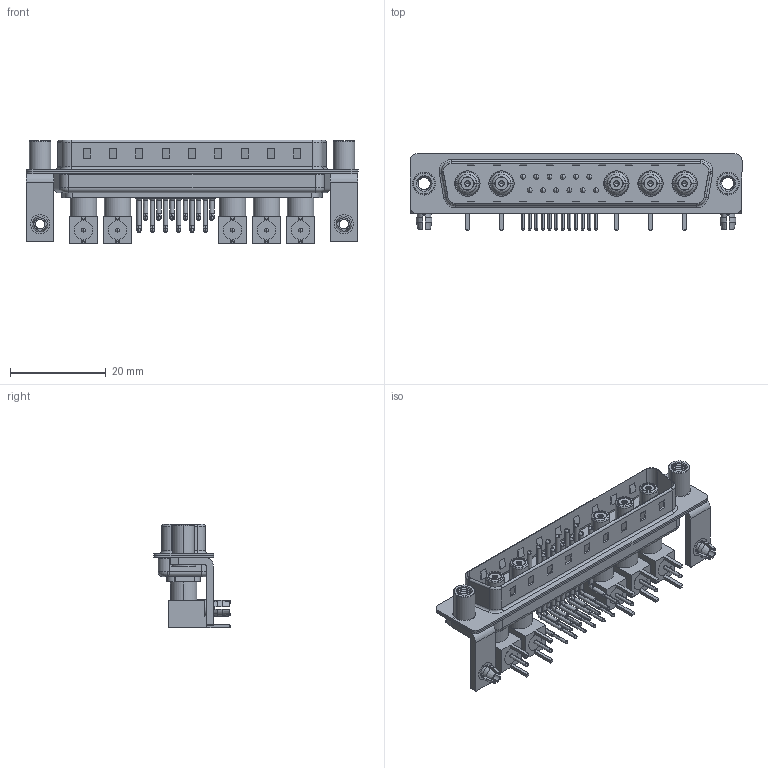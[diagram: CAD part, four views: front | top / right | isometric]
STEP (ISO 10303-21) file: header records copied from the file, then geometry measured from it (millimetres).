
FILE_DESCRIPTION (( 'STEP AP203' ), '1' );
FILE_NAME ('629-17W5240-7ND.STEP', '2022-05-15T00:04:30', ( '' ), ( '' ), 'SwSTEP 2.0', 'SolidWorks 2020', '' );
FILE_SCHEMA (( 'CONFIG_CONTROL_DESIGN' ));
Length unit declared in the file: millimetre
Products named in the file (21): 629Combo Stabilizer Bracket; 629Combo Contact Row 2; 629Combo Shell Front_37 Contacts; Socket_RA; Insulator RA Pin; 629-17W5240-7ND; Co-Ax Jack Assy_RA; Insulator Socket; 629Combo Threaded Standoff_D; Co-Ax Jack_RA PC Tail; 629Combo Housing_17W5; 629Combo Contact Row 1; Locking Collar; 629Combo Shell Rear_37 Contacts; 629Combo Board Lock; RA Back Shell; Insulator Socket 2
Assembly tree (61 placements, depth 3):
  629-17W5240-7ND
    629Combo Housing_17W5
    629Combo Shell Rear_37 Contacts
    629Combo Shell Front_37 Contacts
    629Combo Stabilizer Bracket  x2
    629Combo Board Lock  x2
    629Combo Threaded Standoff_D  x2
    Co-Ax Jack Assy_RA
      Co-Ax Jack_RA PC Tail
      Insulator Socket
      Insulator Socket 2
      Locking Collar
      Socket_RA
      RA Back Shell
      Insulator RA Pin
    Co-Ax Jack Assy_RA
      Co-Ax Jack_RA PC Tail
      Insulator Socket
      Insulator Socket 2
      Locking Collar
      Socket_RA
      RA Back Shell
      Insulator RA Pin
    Co-Ax Jack Assy_RA
      Co-Ax Jack_RA PC Tail
      Insulator Socket
      Insulator Socket 2
      Locking Collar
      Socket_RA
      RA Back Shell
      Insulator RA Pin
    Co-Ax Jack Assy_RA
      Co-Ax Jack_RA PC Tail
      Insulator Socket
      Insulator Socket 2
      Locking Collar
      Socket_RA
      RA Back Shell
      Insulator RA Pin
    Co-Ax Jack Assy_RA
      Co-Ax Jack_RA PC Tail
      Insulator Socket
      Insulator Socket 2
      Locking Collar
      Socket_RA
      RA Back Shell
      Insulator RA Pin
    629Combo Contact Row 1  x6
    629Combo Contact Row 2  x6
Bounding box: 69.4 x 16 x 21.71 mm (x, y, z)
Volume: 5711 mm3; surface area: 15345.9 mm2
Topology: 56 solids, 56 shells, 2682 faces, 7028 edges, 4505 vertices
Faces by surface type: plane 1326, cylinder 1012, cone 171, bspline 83, torus 80, sphere 10
Entity records: 34830 total; most frequent: CARTESIAN_POINT 7790, DIRECTION 5156, ORIENTED_EDGE 4816, EDGE_CURVE 2408, AXIS2_PLACEMENT_3D 1865, VERTEX_POINT 1552, LINE 1426, VECTOR 1426
